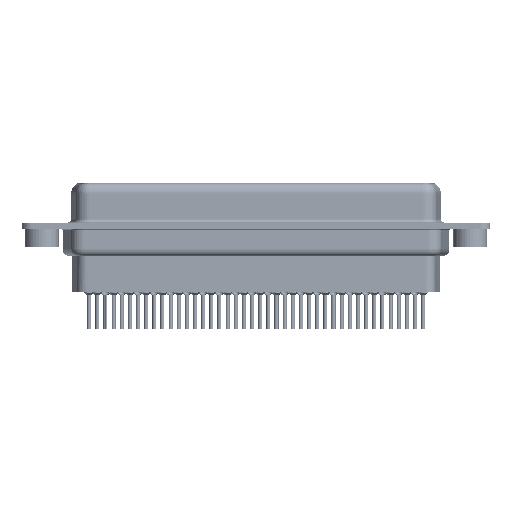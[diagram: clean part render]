
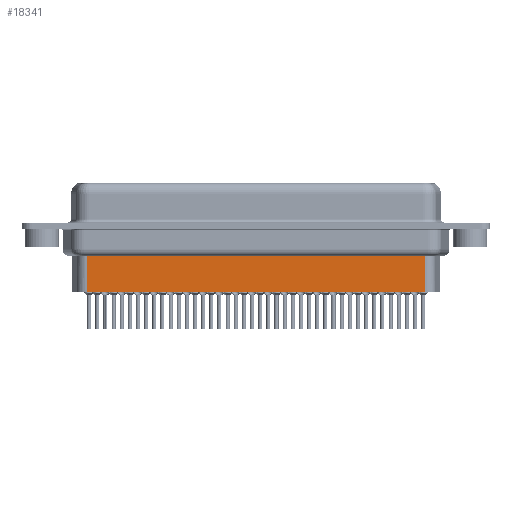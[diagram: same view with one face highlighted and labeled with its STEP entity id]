
A CAD part, front view. The second image highlights one B-rep face of the part: STEP entity #18341.
In plain terms, the highlighted planar face has unit normal (0, -1, 0).
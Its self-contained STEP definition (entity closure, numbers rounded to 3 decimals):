
#1769 = LINE ( 'NONE', #19858, #8862 ) ;
#1845 = CARTESIAN_POINT ( 'NONE',  ( 6.706, -3.5, -9.85 ) ) ;
#3004 = ORIENTED_EDGE ( 'NONE', *, *, #31693, .F. ) ;
#5555 = DIRECTION ( 'NONE',  ( 0., 0., -1. ) ) ;
#8862 = VECTOR ( 'NONE', #8924, 1000. ) ;
#8924 = DIRECTION ( 'NONE',  ( -1., 0., 0. ) ) ;
#9085 = EDGE_CURVE ( 'NONE', #27543, #30937, #16059, .T. ) ;
#9816 = LINE ( 'NONE', #42135, #45461 ) ;
#14013 = ORIENTED_EDGE ( 'NONE', *, *, #9085, .F. ) ;
#14490 = DIRECTION ( 'NONE',  ( 1., 0., 0. ) ) ;
#15846 = CARTESIAN_POINT ( 'NONE',  ( 6.459, -3.5, -4.097 ) ) ;
#16059 = LINE ( 'NONE', #26977, #35927 ) ;
#16071 = DIRECTION ( 'NONE',  ( -1., 0., 0. ) ) ;
#17825 = CARTESIAN_POINT ( 'NONE',  ( 6.706, -3.5, -3.1 ) ) ;
#18341 = ADVANCED_FACE ( 'NONE', ( #38521 ), #39924, .T. ) ;
#18722 = VERTEX_POINT ( 'NONE', #1845 ) ;
#19858 = CARTESIAN_POINT ( 'NONE',  ( 6.706, -3.5, -9.85 ) ) ;
#21460 = AXIS2_PLACEMENT_3D ( 'NONE', #17825, #25411, #14490 ) ;
#22998 = VECTOR ( 'NONE', #16071, 1000. ) ;
#24321 = VERTEX_POINT ( 'NONE', #25344 ) ;
#25344 = CARTESIAN_POINT ( 'NONE',  ( 6.706, -3.5, -4.097 ) ) ;
#25411 = DIRECTION ( 'NONE',  ( 0., -1., 0. ) ) ;
#26692 = CARTESIAN_POINT ( 'NONE',  ( 56.794, -3.5, -9.85 ) ) ;
#26977 = CARTESIAN_POINT ( 'NONE',  ( 56.794, -3.5, -3.1 ) ) ;
#27543 = VERTEX_POINT ( 'NONE', #30063 ) ;
#27900 = DIRECTION ( 'NONE',  ( 0., 0., -1. ) ) ;
#28942 = ORIENTED_EDGE ( 'NONE', *, *, #41295, .T. ) ;
#30063 = CARTESIAN_POINT ( 'NONE',  ( 56.794, -3.5, -4.097 ) ) ;
#30937 = VERTEX_POINT ( 'NONE', #26692 ) ;
#31693 = EDGE_CURVE ( 'NONE', #30937, #18722, #1769, .T. ) ;
#33896 = LINE ( 'NONE', #15846, #22998 ) ;
#35927 = VECTOR ( 'NONE', #5555, 1000. ) ;
#38521 = FACE_OUTER_BOUND ( 'NONE', #46934, .T. ) ;
#39924 = PLANE ( 'NONE',  #21460 ) ;
#40757 = ORIENTED_EDGE ( 'NONE', *, *, #46087, .T. ) ;
#41295 = EDGE_CURVE ( 'NONE', #24321, #18722, #9816, .T. ) ;
#42135 = CARTESIAN_POINT ( 'NONE',  ( 6.706, -3.5, -3.1 ) ) ;
#45461 = VECTOR ( 'NONE', #27900, 1000. ) ;
#46087 = EDGE_CURVE ( 'NONE', #27543, #24321, #33896, .T. ) ;
#46934 = EDGE_LOOP ( 'NONE', ( #14013, #40757, #28942, #3004 ) ) ;
